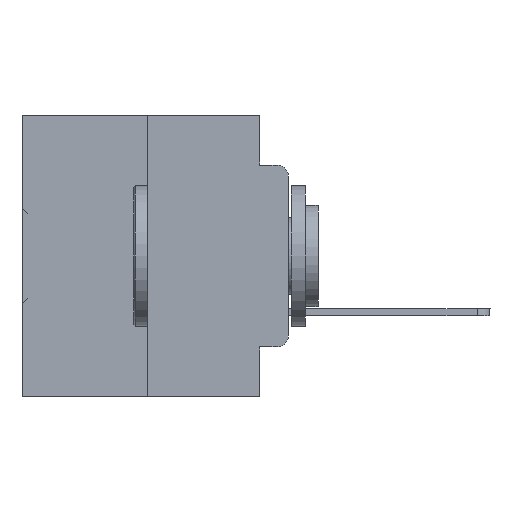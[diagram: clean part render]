
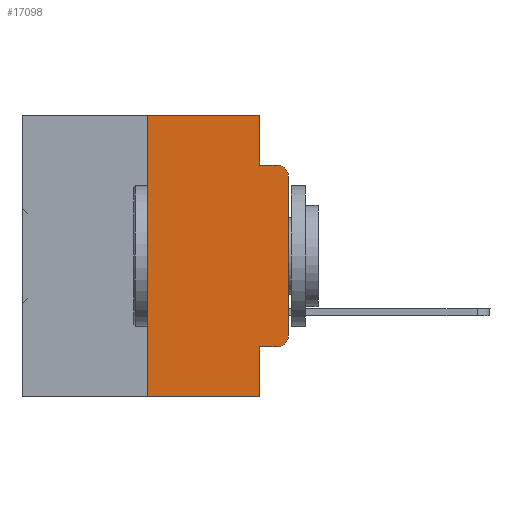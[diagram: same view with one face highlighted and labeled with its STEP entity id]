
A CAD part, left-side view. The second image highlights one B-rep face of the part: STEP entity #17098.
In plain terms, the highlighted planar face has unit normal (-1, 0, 0).
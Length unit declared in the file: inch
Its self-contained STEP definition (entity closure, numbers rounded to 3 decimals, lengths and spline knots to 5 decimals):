
#543 = CARTESIAN_POINT ( 'NONE',  ( 0., 0.25, 0. ) ) ;
#832 = EDGE_CURVE ( 'NONE', #13071, #30364, #25553, .T. ) ;
#1231 = EDGE_CURVE ( 'NONE', #32587, #11122, #5436, .T. ) ;
#1316 = AXIS2_PLACEMENT_3D ( 'NONE', #31716, #34478, #14670 ) ;
#2233 = PLANE ( 'NONE',  #16995 ) ;
#2674 = AXIS2_PLACEMENT_3D ( 'NONE', #12825, #21524, #13206 ) ;
#3361 = VECTOR ( 'NONE', #12090, 39.37008 ) ;
#3393 = VECTOR ( 'NONE', #29140, 39.37008 ) ;
#3594 = VECTOR ( 'NONE', #8052, 39.37008 ) ;
#4020 = CARTESIAN_POINT ( 'NONE',  ( 0., 0., -0.1085 ) ) ;
#4122 = CARTESIAN_POINT ( 'NONE',  ( 0., 0.25, -0.5 ) ) ;
#4750 = VECTOR ( 'NONE', #24025, 39.37008 ) ;
#5157 = FACE_OUTER_BOUND ( 'NONE', #33288, .T. ) ;
#5436 = LINE ( 'NONE', #13640, #3594 ) ;
#5649 = CARTESIAN_POINT ( 'NONE',  ( 0., 0.051, -0.0885 ) ) ;
#6099 = LINE ( 'NONE', #35974, #4750 ) ;
#6667 = ORIENTED_EDGE ( 'NONE', *, *, #27377, .T. ) ;
#6697 = DIRECTION ( 'NONE',  ( 0., 0., -1. ) ) ;
#6933 = CARTESIAN_POINT ( 'NONE',  ( 0., 0.051, 0. ) ) ;
#6994 = CARTESIAN_POINT ( 'NONE',  ( 0., 0.051, -0.4115 ) ) ;
#8052 = DIRECTION ( 'NONE',  ( 0., -1., 0. ) ) ;
#8630 = DIRECTION ( 'NONE',  ( 0., -1., 0. ) ) ;
#8805 = CARTESIAN_POINT ( 'NONE',  ( 0., 0.473, 0. ) ) ;
#9844 = DIRECTION ( 'NONE',  ( 1., 0., 0. ) ) ;
#11038 = VECTOR ( 'NONE', #32907, 39.37008 ) ;
#11122 = VERTEX_POINT ( 'NONE', #33392 ) ;
#11147 = EDGE_CURVE ( 'NONE', #32587, #15537, #23039, .T. ) ;
#11402 = ORIENTED_EDGE ( 'NONE', *, *, #16620, .F. ) ;
#11668 = EDGE_CURVE ( 'NONE', #15214, #36856, #35602, .T. ) ;
#12090 = DIRECTION ( 'NONE',  ( 0., 0., 1. ) ) ;
#12234 = VECTOR ( 'NONE', #6697, 39.37008 ) ;
#12825 = CARTESIAN_POINT ( 'NONE',  ( 0., 0.02, -0.1085 ) ) ;
#13071 = VERTEX_POINT ( 'NONE', #14448 ) ;
#13206 = DIRECTION ( 'NONE',  ( 0., 0., -1. ) ) ;
#13640 = CARTESIAN_POINT ( 'NONE',  ( 0., 0.051, -0.4115 ) ) ;
#13674 = LINE ( 'NONE', #35409, #12234 ) ;
#13961 = CIRCLE ( 'NONE', #1316, 0.02 ) ;
#14448 = CARTESIAN_POINT ( 'NONE',  ( 0., 0.051, -0.0885 ) ) ;
#14670 = DIRECTION ( 'NONE',  ( 0., 0., -1. ) ) ;
#15214 = VERTEX_POINT ( 'NONE', #15541 ) ;
#15537 = VERTEX_POINT ( 'NONE', #21582 ) ;
#15541 = CARTESIAN_POINT ( 'NONE',  ( 0., 0., -0.3915 ) ) ;
#15558 = ORIENTED_EDGE ( 'NONE', *, *, #832, .F. ) ;
#15932 = VERTEX_POINT ( 'NONE', #4122 ) ;
#15955 = EDGE_CURVE ( 'NONE', #15932, #15537, #6099, .T. ) ;
#16620 = EDGE_CURVE ( 'NONE', #34514, #26040, #35635, .T. ) ;
#16685 = ORIENTED_EDGE ( 'NONE', *, *, #17984, .T. ) ;
#16705 = CARTESIAN_POINT ( 'NONE',  ( 0., 0.473, 0. ) ) ;
#16995 = AXIS2_PLACEMENT_3D ( 'NONE', #16705, #9844, #29698 ) ;
#17098 = ADVANCED_FACE ( 'NONE', ( #5157 ), #2233, .F. ) ;
#17319 = LINE ( 'NONE', #543, #37045 ) ;
#17495 = ORIENTED_EDGE ( 'NONE', *, *, #19065, .F. ) ;
#17984 = EDGE_CURVE ( 'NONE', #36856, #30364, #22479, .T. ) ;
#19065 = EDGE_CURVE ( 'NONE', #26040, #13071, #13674, .T. ) ;
#21278 = ORIENTED_EDGE ( 'NONE', *, *, #1231, .T. ) ;
#21524 = DIRECTION ( 'NONE',  ( -1., 0., 0. ) ) ;
#21582 = CARTESIAN_POINT ( 'NONE',  ( 0., 0.051, -0.5 ) ) ;
#22479 = CIRCLE ( 'NONE', #2674, 0.02 ) ;
#23039 = LINE ( 'NONE', #29552, #3393 ) ;
#23264 = VECTOR ( 'NONE', #8630, 39.37008 ) ;
#24025 = DIRECTION ( 'NONE',  ( 0., -1., 0. ) ) ;
#24143 = ORIENTED_EDGE ( 'NONE', *, *, #15955, .T. ) ;
#25553 = LINE ( 'NONE', #5649, #23264 ) ;
#26040 = VERTEX_POINT ( 'NONE', #6933 ) ;
#27377 = EDGE_CURVE ( 'NONE', #11122, #15214, #13961, .T. ) ;
#27653 = ORIENTED_EDGE ( 'NONE', *, *, #11147, .F. ) ;
#29140 = DIRECTION ( 'NONE',  ( 0., 0., -1. ) ) ;
#29552 = CARTESIAN_POINT ( 'NONE',  ( 0., 0.051, 0. ) ) ;
#29626 = EDGE_CURVE ( 'NONE', #15932, #34514, #17319, .T. ) ;
#29698 = DIRECTION ( 'NONE',  ( 0., 0., -1. ) ) ;
#30364 = VERTEX_POINT ( 'NONE', #33162 ) ;
#31716 = CARTESIAN_POINT ( 'NONE',  ( 0., 0.02, -0.3915 ) ) ;
#32330 = CARTESIAN_POINT ( 'NONE',  ( 0., 0.25, 0. ) ) ;
#32376 = CARTESIAN_POINT ( 'NONE',  ( 0., 0., 0. ) ) ;
#32587 = VERTEX_POINT ( 'NONE', #6994 ) ;
#32907 = DIRECTION ( 'NONE',  ( 0., -1., 0. ) ) ;
#32954 = ORIENTED_EDGE ( 'NONE', *, *, #11668, .T. ) ;
#33162 = CARTESIAN_POINT ( 'NONE',  ( 0., 0.02, -0.0885 ) ) ;
#33288 = EDGE_LOOP ( 'NONE', ( #32954, #16685, #15558, #17495, #11402, #34465, #24143, #27653, #21278, #6667 ) ) ;
#33392 = CARTESIAN_POINT ( 'NONE',  ( 0., 0.02, -0.4115 ) ) ;
#34450 = DIRECTION ( 'NONE',  ( 0., 0., 1. ) ) ;
#34465 = ORIENTED_EDGE ( 'NONE', *, *, #29626, .F. ) ;
#34478 = DIRECTION ( 'NONE',  ( -1., 0., 0. ) ) ;
#34514 = VERTEX_POINT ( 'NONE', #32330 ) ;
#35409 = CARTESIAN_POINT ( 'NONE',  ( 0., 0.051, 0. ) ) ;
#35602 = LINE ( 'NONE', #32376, #3361 ) ;
#35635 = LINE ( 'NONE', #8805, #11038 ) ;
#35974 = CARTESIAN_POINT ( 'NONE',  ( 0., 0.473, -0.5 ) ) ;
#36856 = VERTEX_POINT ( 'NONE', #4020 ) ;
#37045 = VECTOR ( 'NONE', #34450, 39.37008 ) ;
